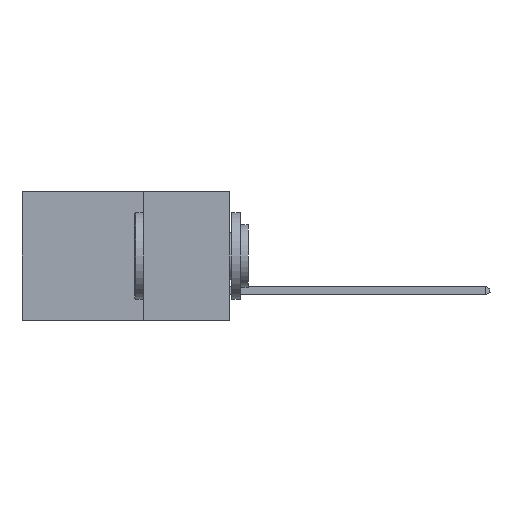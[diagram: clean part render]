
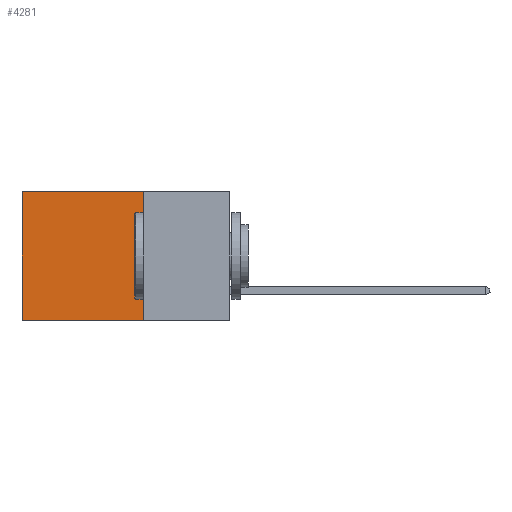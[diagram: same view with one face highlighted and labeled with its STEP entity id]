
A CAD part, left-side view. The second image highlights one B-rep face of the part: STEP entity #4281.
In plain terms, the highlighted planar face has unit normal (-1, 0, 0).
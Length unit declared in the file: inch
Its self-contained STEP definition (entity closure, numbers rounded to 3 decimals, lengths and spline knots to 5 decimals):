
#1016 = EDGE_CURVE ( 'NONE', #8131, #11670, #12360, .T. ) ;
#1077 = VECTOR ( 'NONE', #11558, 39.37008 ) ;
#2334 = ORIENTED_EDGE ( 'NONE', *, *, #22136, .F. ) ;
#3589 = VECTOR ( 'NONE', #17831, 39.37008 ) ;
#4197 = CARTESIAN_POINT ( 'NONE',  ( 0.298, 0.25, 0. ) ) ;
#4281 = ADVANCED_FACE ( 'NONE', ( #20517 ), #18906, .F. ) ;
#4368 = VECTOR ( 'NONE', #19483, 39.37008 ) ;
#6491 = VECTOR ( 'NONE', #11803, 39.37008 ) ;
#6847 = CARTESIAN_POINT ( 'NONE',  ( 0.298, 0.6, -0.37 ) ) ;
#7198 = CARTESIAN_POINT ( 'NONE',  ( 0.298, 0.25, 0. ) ) ;
#7543 = DIRECTION ( 'NONE',  ( 0., 0., -1. ) ) ;
#7805 = EDGE_CURVE ( 'NONE', #8131, #18554, #9062, .T. ) ;
#8131 = VERTEX_POINT ( 'NONE', #7198 ) ;
#9062 = LINE ( 'NONE', #21303, #1077 ) ;
#9338 = CARTESIAN_POINT ( 'NONE',  ( 0.298, 0.25, -0.37 ) ) ;
#9629 = CARTESIAN_POINT ( 'NONE',  ( 0.298, 0.25, 0. ) ) ;
#9905 = VERTEX_POINT ( 'NONE', #6847 ) ;
#10625 = CARTESIAN_POINT ( 'NONE',  ( 0.298, 0.6, 0. ) ) ;
#11558 = DIRECTION ( 'NONE',  ( 0., 0., -1. ) ) ;
#11670 = VERTEX_POINT ( 'NONE', #10625 ) ;
#11803 = DIRECTION ( 'NONE',  ( 0., 0., -1. ) ) ;
#12360 = LINE ( 'NONE', #4197, #4368 ) ;
#13754 = CARTESIAN_POINT ( 'NONE',  ( 0.298, 0.6, 0. ) ) ;
#14796 = LINE ( 'NONE', #13754, #6491 ) ;
#15491 = EDGE_LOOP ( 'NONE', ( #17861, #2334, #16834, #20871 ) ) ;
#16834 = ORIENTED_EDGE ( 'NONE', *, *, #7805, .F. ) ;
#17249 = DIRECTION ( 'NONE',  ( 1., 0., 0. ) ) ;
#17831 = DIRECTION ( 'NONE',  ( 0., 1., 0. ) ) ;
#17861 = ORIENTED_EDGE ( 'NONE', *, *, #22866, .T. ) ;
#18554 = VERTEX_POINT ( 'NONE', #9338 ) ;
#18906 = PLANE ( 'NONE',  #20521 ) ;
#19483 = DIRECTION ( 'NONE',  ( 0., 1., 0. ) ) ;
#20517 = FACE_OUTER_BOUND ( 'NONE', #15491, .T. ) ;
#20521 = AXIS2_PLACEMENT_3D ( 'NONE', #9629, #17249, #7543 ) ;
#20871 = ORIENTED_EDGE ( 'NONE', *, *, #1016, .T. ) ;
#21303 = CARTESIAN_POINT ( 'NONE',  ( 0.298, 0.25, 0. ) ) ;
#22136 = EDGE_CURVE ( 'NONE', #18554, #9905, #22834, .T. ) ;
#22834 = LINE ( 'NONE', #23546, #3589 ) ;
#22866 = EDGE_CURVE ( 'NONE', #11670, #9905, #14796, .T. ) ;
#23546 = CARTESIAN_POINT ( 'NONE',  ( 0.298, 0.25, -0.37 ) ) ;
